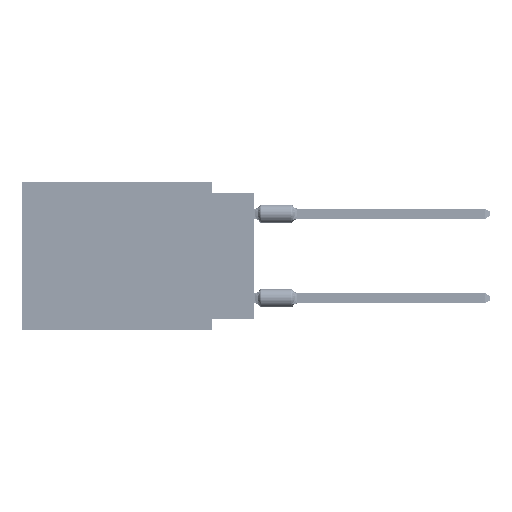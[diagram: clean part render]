
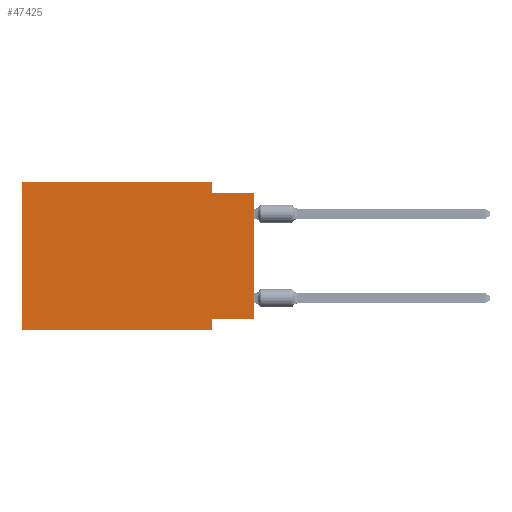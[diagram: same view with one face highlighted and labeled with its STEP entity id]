
A CAD part, left-side view. The second image highlights one B-rep face of the part: STEP entity #47425.
In plain terms, the highlighted planar face has unit normal (-1, 0, 0).
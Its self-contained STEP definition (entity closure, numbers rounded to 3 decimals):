
#1194 = VECTOR ( 'NONE', #38782, 1000. ) ;
#2339 = VECTOR ( 'NONE', #73136, 1000. ) ;
#3557 = ORIENTED_EDGE ( 'NONE', *, *, #32543, .F. ) ;
#3833 = VECTOR ( 'NONE', #44601, 1000. ) ;
#4623 = EDGE_CURVE ( 'NONE', #13065, #9796, #36863, .T. ) ;
#4831 = VERTEX_POINT ( 'NONE', #58406 ) ;
#6042 = CARTESIAN_POINT ( 'NONE',  ( 0., 13.97, 0. ) ) ;
#7458 = VECTOR ( 'NONE', #63557, 1000. ) ;
#8543 = VERTEX_POINT ( 'NONE', #23202 ) ;
#8835 = EDGE_CURVE ( 'NONE', #9273, #4831, #54881, .T. ) ;
#9273 = VERTEX_POINT ( 'NONE', #54797 ) ;
#9796 = VERTEX_POINT ( 'NONE', #64528 ) ;
#11606 = ORIENTED_EDGE ( 'NONE', *, *, #47635, .F. ) ;
#11688 = EDGE_CURVE ( 'NONE', #28344, #14891, #39040, .T. ) ;
#13065 = VERTEX_POINT ( 'NONE', #35649 ) ;
#13575 = CARTESIAN_POINT ( 'NONE',  ( 0., 13.97, 0. ) ) ;
#14891 = VERTEX_POINT ( 'NONE', #56416 ) ;
#15857 = LINE ( 'NONE', #50339, #1194 ) ;
#18687 = FACE_OUTER_BOUND ( 'NONE', #71845, .T. ) ;
#20469 = CARTESIAN_POINT ( 'NONE',  ( 0., 13.97, 0. ) ) ;
#21414 = CARTESIAN_POINT ( 'NONE',  ( 0., 2.54, 0. ) ) ;
#23202 = CARTESIAN_POINT ( 'NONE',  ( 0., 2.54, -8.89 ) ) ;
#24665 = PLANE ( 'NONE',  #39331 ) ;
#27129 = VECTOR ( 'NONE', #31266, 1000. ) ;
#27667 = LINE ( 'NONE', #67569, #65167 ) ;
#27849 = CARTESIAN_POINT ( 'NONE',  ( 0., 2.54, 0. ) ) ;
#28344 = VERTEX_POINT ( 'NONE', #21414 ) ;
#28795 = DIRECTION ( 'NONE',  ( 0., 0., -1. ) ) ;
#29064 = ORIENTED_EDGE ( 'NONE', *, *, #48144, .T. ) ;
#31266 = DIRECTION ( 'NONE',  ( 0., 0., 1. ) ) ;
#32543 = EDGE_CURVE ( 'NONE', #9796, #28344, #64312, .T. ) ;
#35469 = DIRECTION ( 'NONE',  ( 1., 0., 0. ) ) ;
#35533 = ORIENTED_EDGE ( 'NONE', *, *, #56440, .T. ) ;
#35649 = CARTESIAN_POINT ( 'NONE',  ( 0., 13.97, -8.89 ) ) ;
#36863 = LINE ( 'NONE', #20469, #27129 ) ;
#36898 = ORIENTED_EDGE ( 'NONE', *, *, #8835, .F. ) ;
#38782 = DIRECTION ( 'NONE',  ( 0., 0., -1. ) ) ;
#39040 = LINE ( 'NONE', #27849, #3833 ) ;
#39331 = AXIS2_PLACEMENT_3D ( 'NONE', #6042, #35469, #28795 ) ;
#39386 = VECTOR ( 'NONE', #51711, 1000. ) ;
#41167 = CARTESIAN_POINT ( 'NONE',  ( 0., 0., 0. ) ) ;
#44601 = DIRECTION ( 'NONE',  ( 0., 0., -1. ) ) ;
#46012 = VERTEX_POINT ( 'NONE', #67219 ) ;
#47425 = ADVANCED_FACE ( 'NONE', ( #18687 ), #24665, .F. ) ;
#47635 = EDGE_CURVE ( 'NONE', #4831, #8543, #15857, .T. ) ;
#47878 = DIRECTION ( 'NONE',  ( 0., 0., 1. ) ) ;
#48144 = EDGE_CURVE ( 'NONE', #13065, #8543, #56955, .T. ) ;
#50339 = CARTESIAN_POINT ( 'NONE',  ( 0., 2.54, -8.89 ) ) ;
#50997 = ORIENTED_EDGE ( 'NONE', *, *, #58397, .F. ) ;
#51711 = DIRECTION ( 'NONE',  ( 0., -1., 0. ) ) ;
#52817 = ORIENTED_EDGE ( 'NONE', *, *, #11688, .F. ) ;
#53867 = LINE ( 'NONE', #41167, #63688 ) ;
#54797 = CARTESIAN_POINT ( 'NONE',  ( 0., 0., -8.255 ) ) ;
#54881 = LINE ( 'NONE', #60479, #2339 ) ;
#56416 = CARTESIAN_POINT ( 'NONE',  ( 0., 2.54, -0.635 ) ) ;
#56440 = EDGE_CURVE ( 'NONE', #9273, #46012, #53867, .T. ) ;
#56955 = LINE ( 'NONE', #63290, #39386 ) ;
#58397 = EDGE_CURVE ( 'NONE', #14891, #46012, #27667, .T. ) ;
#58406 = CARTESIAN_POINT ( 'NONE',  ( 0., 2.54, -8.255 ) ) ;
#60479 = CARTESIAN_POINT ( 'NONE',  ( 0., 0., -8.255 ) ) ;
#61979 = DIRECTION ( 'NONE',  ( 0., -1., 0. ) ) ;
#63290 = CARTESIAN_POINT ( 'NONE',  ( 0., 13.97, -8.89 ) ) ;
#63557 = DIRECTION ( 'NONE',  ( 0., -1., 0. ) ) ;
#63688 = VECTOR ( 'NONE', #47878, 1000. ) ;
#64312 = LINE ( 'NONE', #13575, #7458 ) ;
#64528 = CARTESIAN_POINT ( 'NONE',  ( 0., 13.97, 0. ) ) ;
#65167 = VECTOR ( 'NONE', #61979, 1000. ) ;
#67219 = CARTESIAN_POINT ( 'NONE',  ( 0., 0., -0.635 ) ) ;
#67569 = CARTESIAN_POINT ( 'NONE',  ( 0., 0., -0.635 ) ) ;
#67673 = ORIENTED_EDGE ( 'NONE', *, *, #4623, .F. ) ;
#71845 = EDGE_LOOP ( 'NONE', ( #35533, #50997, #52817, #3557, #67673, #29064, #11606, #36898 ) ) ;
#73136 = DIRECTION ( 'NONE',  ( 0., 1., 0. ) ) ;
